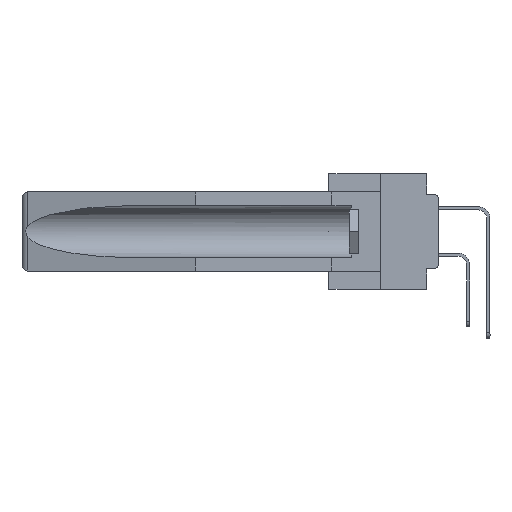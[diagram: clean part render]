
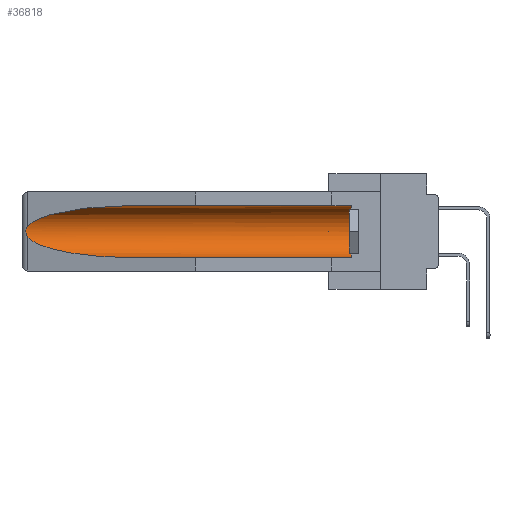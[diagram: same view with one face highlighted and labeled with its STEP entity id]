
A CAD part, left-side view. The second image highlights one B-rep face of the part: STEP entity #36818.
In plain terms, the highlighted cylindrical face has radius 2.857 mm (diameter 5.715 mm), a partial arc.
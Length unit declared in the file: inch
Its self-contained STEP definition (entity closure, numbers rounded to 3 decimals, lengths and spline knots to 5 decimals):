
#2297 = DIRECTION ( 'NONE',  ( 0., 0., 1. ) ) ;
#2899 = CARTESIAN_POINT ( 'NONE',  ( 0.26597, 1.5296, -0.19026 ) ) ;
#3554 = EDGE_CURVE ( 'NONE', #40921, #21981, #24317, .T. ) ;
#5666 = LINE ( 'NONE', #18357, #18355 ) ;
#5717 = CARTESIAN_POINT ( 'NONE',  ( 0.21114, 1.30732, -0.059 ) ) ;
#5847 = CARTESIAN_POINT ( 'NONE',  ( 0.2673, 1.5327, -0.16383 ) ) ;
#6647 = CIRCLE ( 'NONE', #13965, 0.1125 ) ;
#6816 = DIRECTION ( 'NONE',  ( 0., 1., 0. ) ) ;
#7182 = ORIENTED_EDGE ( 'NONE', *, *, #39101, .F. ) ;
#8006 = EDGE_LOOP ( 'NONE', ( #13500, #20919, #12218, #7182, #11596, #30592 ) ) ;
#8118 = CARTESIAN_POINT ( 'NONE',  ( 0.155, 1.07973, -0.284 ) ) ;
#8770 = LINE ( 'NONE', #24429, #11663 ) ;
#8798 = CARTESIAN_POINT ( 'NONE',  ( 0.26537, 1.52718, -0.19328 ) ) ;
#9304 = B_SPLINE_CURVE_WITH_KNOTS ( 'NONE', 3,
 ( #34442, #40927, #31317, #5847, #38389, #38185, #9792, #27976, #2899, #31514 ),
 .UNSPECIFIED., .F., .F.,
 ( 4, 2, 2, 2, 4 ),
 ( 0., 0.00029, 0.00058, 0.00087, 0.00117 ),
 .UNSPECIFIED. ) ;
#9792 = CARTESIAN_POINT ( 'NONE',  ( 0.2673, 1.53269, -0.17917 ) ) ;
#11562 = CARTESIAN_POINT ( 'NONE',  ( 0.26537, 1.52718, -0.14972 ) ) ;
#11596 = ORIENTED_EDGE ( 'NONE', *, *, #21359, .T. ) ;
#11663 = VECTOR ( 'NONE', #6816, 39.37008 ) ;
#12218 = ORIENTED_EDGE ( 'NONE', *, *, #16761, .T. ) ;
#12536 = DIRECTION ( 'NONE',  ( 0., 0., 1. ) ) ;
#13500 = ORIENTED_EDGE ( 'NONE', *, *, #3554, .T. ) ;
#13965 = AXIS2_PLACEMENT_3D ( 'NONE', #34463, #28400, #12536 ) ;
#14371 = CARTESIAN_POINT ( 'NONE',  ( 0.21114, 1.30732, -0.284 ) ) ;
#14815 = CARTESIAN_POINT ( 'NONE',  ( 0.155, 0.126, -0.059 ) ) ;
#14853 = DIRECTION ( 'NONE',  ( 0., 1., 0. ) ) ;
#15877 = VERTEX_POINT ( 'NONE', #29536 ) ;
#16761 = EDGE_CURVE ( 'NONE', #31365, #15877, #24572, .T. ) ;
#18355 = VECTOR ( 'NONE', #14853, 39.37008 ) ;
#18357 = CARTESIAN_POINT ( 'NONE',  ( 0.155, -0.30754, -0.059 ) ) ;
#20189 = CARTESIAN_POINT ( 'NONE',  ( 0.155, 0.126, -0.284 ) ) ;
#20919 = ORIENTED_EDGE ( 'NONE', *, *, #29056, .T. ) ;
#21359 = EDGE_CURVE ( 'NONE', #37105, #31668, #6647, .T. ) ;
#21677 = CYLINDRICAL_SURFACE ( 'NONE', #38850, 0.1125 ) ;
#21886 = CARTESIAN_POINT ( 'NONE',  ( 0.155, -0.30754, -0.1715 ) ) ;
#21981 = VERTEX_POINT ( 'NONE', #11562 ) ;
#24317 =( BOUNDED_CURVE ( )  B_SPLINE_CURVE ( 3, ( #37867, #5717, #34916, #28250 ),
 .UNSPECIFIED., .F., .F. ) 
 B_SPLINE_CURVE_WITH_KNOTS ( ( 4, 4 ),
 ( 4.71239, 6.08839 ),
 .UNSPECIFIED. ) 
 CURVE ( )  GEOMETRIC_REPRESENTATION_ITEM ( )  RATIONAL_B_SPLINE_CURVE ( ( 1., 0.848, 0.848, 1. ) ) 
 REPRESENTATION_ITEM ( '' )  );
#24429 = CARTESIAN_POINT ( 'NONE',  ( 0.155, -0.30754, -0.284 ) ) ;
#24572 =( BOUNDED_CURVE ( )  B_SPLINE_CURVE ( 3, ( #30459, #30246, #14371, #8118 ),
 .UNSPECIFIED., .F., .F. ) 
 B_SPLINE_CURVE_WITH_KNOTS ( ( 4, 4 ),
 ( 0.1948, 1.5708 ),
 .UNSPECIFIED. ) 
 CURVE ( )  GEOMETRIC_REPRESENTATION_ITEM ( )  RATIONAL_B_SPLINE_CURVE ( ( 1., 0.848, 0.848, 1. ) ) 
 REPRESENTATION_ITEM ( '' )  );
#25036 = DIRECTION ( 'NONE',  ( 0., 1., 0. ) ) ;
#27976 = CARTESIAN_POINT ( 'NONE',  ( 0.26655, 1.53094, -0.18657 ) ) ;
#28250 = CARTESIAN_POINT ( 'NONE',  ( 0.26537, 1.52718, -0.14972 ) ) ;
#28400 = DIRECTION ( 'NONE',  ( 0., -1., 0. ) ) ;
#29056 = EDGE_CURVE ( 'NONE', #21981, #31365, #9304, .T. ) ;
#29536 = CARTESIAN_POINT ( 'NONE',  ( 0.155, 1.07973, -0.284 ) ) ;
#29929 = EDGE_CURVE ( 'NONE', #31668, #40921, #5666, .T. ) ;
#30246 = CARTESIAN_POINT ( 'NONE',  ( 0.25451, 1.48313, -0.24835 ) ) ;
#30459 = CARTESIAN_POINT ( 'NONE',  ( 0.26537, 1.52718, -0.19328 ) ) ;
#30592 = ORIENTED_EDGE ( 'NONE', *, *, #29929, .T. ) ;
#31317 = CARTESIAN_POINT ( 'NONE',  ( 0.26654, 1.53092, -0.15636 ) ) ;
#31365 = VERTEX_POINT ( 'NONE', #8798 ) ;
#31514 = CARTESIAN_POINT ( 'NONE',  ( 0.26537, 1.52718, -0.19328 ) ) ;
#31668 = VERTEX_POINT ( 'NONE', #14815 ) ;
#34442 = CARTESIAN_POINT ( 'NONE',  ( 0.26537, 1.52718, -0.14972 ) ) ;
#34463 = CARTESIAN_POINT ( 'NONE',  ( 0.155, 0.126, -0.1715 ) ) ;
#34916 = CARTESIAN_POINT ( 'NONE',  ( 0.25451, 1.48313, -0.09465 ) ) ;
#36818 = ADVANCED_FACE ( 'NONE', ( #41133 ), #21677, .F. ) ;
#37105 = VERTEX_POINT ( 'NONE', #20189 ) ;
#37867 = CARTESIAN_POINT ( 'NONE',  ( 0.155, 1.07973, -0.059 ) ) ;
#38185 = CARTESIAN_POINT ( 'NONE',  ( 0.2675, 1.53308, -0.17534 ) ) ;
#38389 = CARTESIAN_POINT ( 'NONE',  ( 0.2675, 1.53308, -0.16763 ) ) ;
#38850 = AXIS2_PLACEMENT_3D ( 'NONE', #21886, #25036, #2297 ) ;
#39101 = EDGE_CURVE ( 'NONE', #37105, #15877, #8770, .T. ) ;
#40921 = VERTEX_POINT ( 'NONE', #41086 ) ;
#40927 = CARTESIAN_POINT ( 'NONE',  ( 0.26597, 1.52961, -0.15275 ) ) ;
#41086 = CARTESIAN_POINT ( 'NONE',  ( 0.155, 1.07973, -0.059 ) ) ;
#41133 = FACE_OUTER_BOUND ( 'NONE', #8006, .T. ) ;
